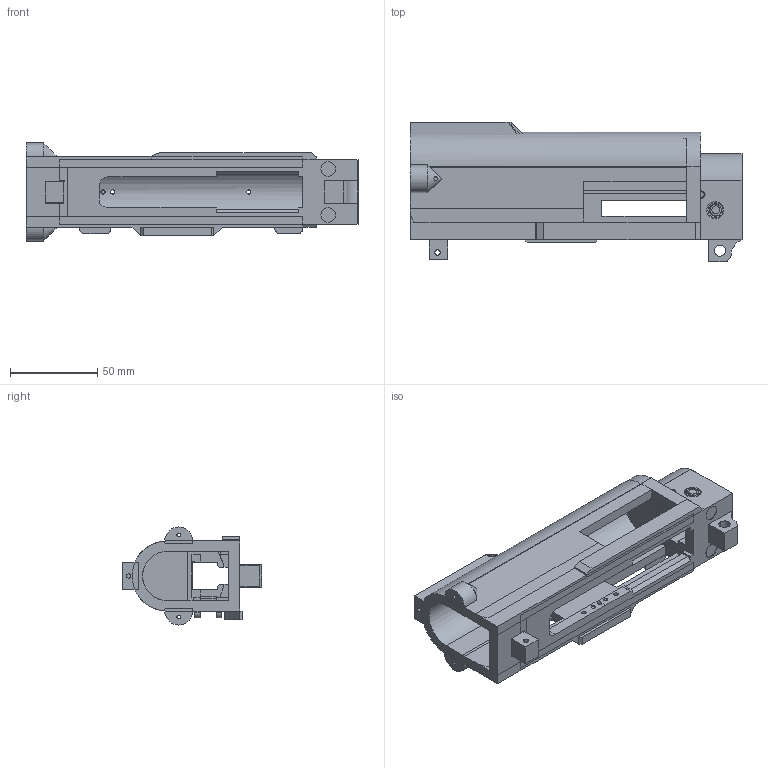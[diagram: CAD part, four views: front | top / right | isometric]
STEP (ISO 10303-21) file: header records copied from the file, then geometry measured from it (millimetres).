
FILE_DESCRIPTION(('FreeCAD Model'),'2;1');
FILE_NAME('ap9 upper pla.step' ,'2018-08-08T20:40:54',('Author'),(''), 'Open CASCADE STEP processor 6.8','FreeCAD','Unknown');
FILE_SCHEMA(('AUTOMOTIVE_DESIGN_CC2 { 1 2 10303 214 -1 1 5 4 }'));
Length unit declared in the file: millimetre
Products named in the file (1): Pocket017
Bounding box: 190.38 x 80.21 x 56.2 mm (x, y, z)
Volume: 192097.1 mm3; surface area: 65416.8 mm2
Topology: 1 solids, 2 shells, 348 faces, 1016 edges, 677 vertices
Faces by surface type: plane 288, cylinder 58, cone 2
Full cylindrical faces by diameter (mm): 2 x1, 2.2 x2, 2.4 x12, 2.6 x2, 8 x1, 8.4 x2
Entity records: 28293 total; most frequent: CARTESIAN_POINT 8650, DIRECTION 3454, LINE 2358, VECTOR 2358, ORIENTED_EDGE 2032, PCURVE 2032, DEFINITIONAL_REPRESENTATION 2032, EDGE_CURVE 1016
